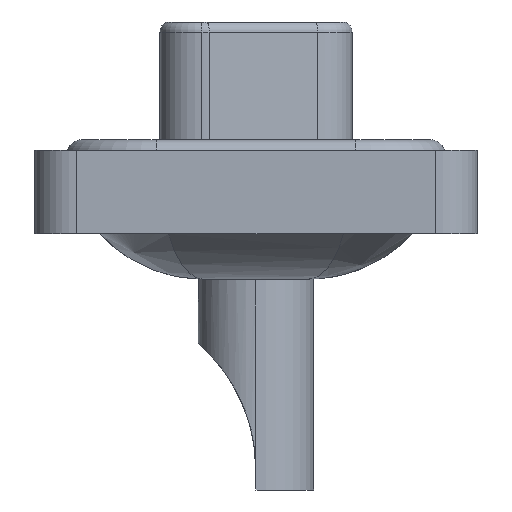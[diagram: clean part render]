
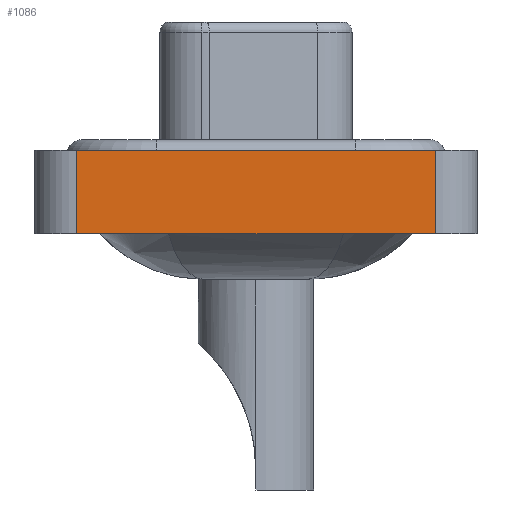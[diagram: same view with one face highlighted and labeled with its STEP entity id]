
A CAD part, left-side view. The second image highlights one B-rep face of the part: STEP entity #1086.
In plain terms, the highlighted planar face has unit normal (-1, 0, 0).
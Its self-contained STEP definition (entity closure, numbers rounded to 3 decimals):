
#632 = DIRECTION ( 'NONE',  ( 0., 0., 1. ) ) ;
#1086 = ADVANCED_FACE ( 'NONE', ( #14660 ), #11586, .T. ) ;
#1317 = VECTOR ( 'NONE', #17360, 1000. ) ;
#1931 = CARTESIAN_POINT ( 'NONE',  ( -7.3, 8.55, -3.6 ) ) ;
#3072 = EDGE_LOOP ( 'NONE', ( #19476, #8138, #12730, #7669 ) ) ;
#3479 = VERTEX_POINT ( 'NONE', #5937 ) ;
#4512 = DIRECTION ( 'NONE',  ( 0., -1., 0. ) ) ;
#4606 = DIRECTION ( 'NONE',  ( 0., -1., 0. ) ) ;
#5606 = CARTESIAN_POINT ( 'NONE',  ( -7.3, -8.55, 0.4 ) ) ;
#5937 = CARTESIAN_POINT ( 'NONE',  ( -7.3, -8.55, -3.6 ) ) ;
#6300 = EDGE_CURVE ( 'NONE', #3479, #16200, #17453, .T. ) ;
#7455 = VERTEX_POINT ( 'NONE', #16977 ) ;
#7669 = ORIENTED_EDGE ( 'NONE', *, *, #17617, .T. ) ;
#7779 = VECTOR ( 'NONE', #4512, 1000. ) ;
#8138 = ORIENTED_EDGE ( 'NONE', *, *, #14334, .F. ) ;
#9684 = EDGE_CURVE ( 'NONE', #7455, #19011, #17238, .T. ) ;
#9860 = CARTESIAN_POINT ( 'NONE',  ( -7.3, -8.55, -3.6 ) ) ;
#11586 = PLANE ( 'NONE',  #14640 ) ;
#12112 = LINE ( 'NONE', #18220, #7779 ) ;
#12271 = VECTOR ( 'NONE', #4606, 1000. ) ;
#12730 = ORIENTED_EDGE ( 'NONE', *, *, #9684, .F. ) ;
#12988 = CARTESIAN_POINT ( 'NONE',  ( -7.3, -8.55, -3.6 ) ) ;
#14334 = EDGE_CURVE ( 'NONE', #19011, #16200, #14798, .T. ) ;
#14640 = AXIS2_PLACEMENT_3D ( 'NONE', #12988, #19180, #17685 ) ;
#14660 = FACE_OUTER_BOUND ( 'NONE', #3072, .T. ) ;
#14798 = LINE ( 'NONE', #16690, #12271 ) ;
#16200 = VERTEX_POINT ( 'NONE', #5606 ) ;
#16690 = CARTESIAN_POINT ( 'NONE',  ( -7.3, -8.55, 0.4 ) ) ;
#16977 = CARTESIAN_POINT ( 'NONE',  ( -7.3, 8.55, -3.6 ) ) ;
#17204 = CARTESIAN_POINT ( 'NONE',  ( -7.3, 8.55, 0.4 ) ) ;
#17238 = LINE ( 'NONE', #1931, #18241 ) ;
#17360 = DIRECTION ( 'NONE',  ( 0., 0., 1. ) ) ;
#17453 = LINE ( 'NONE', #9860, #1317 ) ;
#17617 = EDGE_CURVE ( 'NONE', #7455, #3479, #12112, .T. ) ;
#17685 = DIRECTION ( 'NONE',  ( 0., 0., 1. ) ) ;
#18220 = CARTESIAN_POINT ( 'NONE',  ( -7.3, -8.55, -3.6 ) ) ;
#18241 = VECTOR ( 'NONE', #632, 1000. ) ;
#19011 = VERTEX_POINT ( 'NONE', #17204 ) ;
#19180 = DIRECTION ( 'NONE',  ( -1., 0., 0. ) ) ;
#19476 = ORIENTED_EDGE ( 'NONE', *, *, #6300, .T. ) ;
